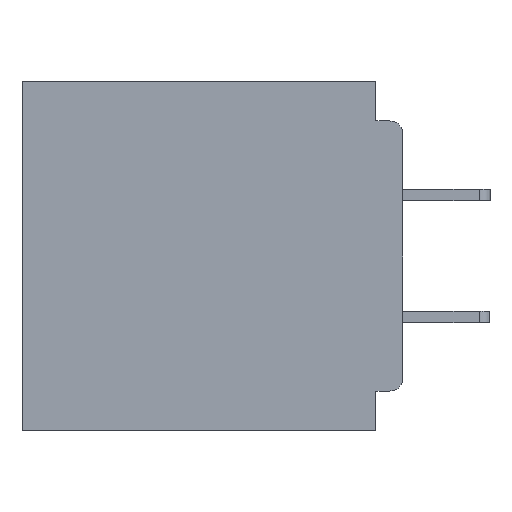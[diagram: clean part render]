
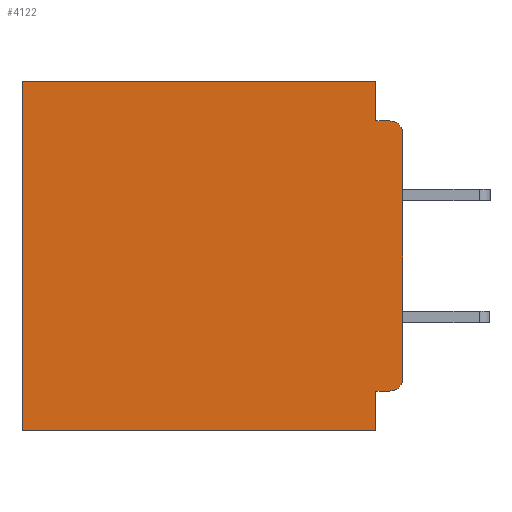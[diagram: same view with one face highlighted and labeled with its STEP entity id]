
A CAD part, left-side view. The second image highlights one B-rep face of the part: STEP entity #4122.
In plain terms, the highlighted planar face has unit normal (-1, 0, 0).
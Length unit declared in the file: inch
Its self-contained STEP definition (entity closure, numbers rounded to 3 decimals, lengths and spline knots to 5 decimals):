
#829 = DIRECTION ( 'NONE',  ( 0., 0., -1. ) ) ;
#1497 = EDGE_CURVE ( 'NONE', #15435, #42395, #46461, .T. ) ;
#2104 = VERTEX_POINT ( 'NONE', #49662 ) ;
#2227 = CARTESIAN_POINT ( 'NONE',  ( 0.3, 0., -0.4 ) ) ;
#4122 = ADVANCED_FACE ( 'NONE', ( #38104 ), #5828, .F. ) ;
#4322 = CARTESIAN_POINT ( 'NONE',  ( 0.3, 0., -0.045 ) ) ;
#4369 = VECTOR ( 'NONE', #24599, 39.37008 ) ;
#4774 = LINE ( 'NONE', #38134, #16652 ) ;
#5394 = CARTESIAN_POINT ( 'NONE',  ( 0.3, 0., -0.4 ) ) ;
#5728 = DIRECTION ( 'NONE',  ( 0., 0., -1. ) ) ;
#5828 = PLANE ( 'NONE',  #31712 ) ;
#6234 = LINE ( 'NONE', #2227, #47389 ) ;
#6326 = VECTOR ( 'NONE', #12518, 39.37008 ) ;
#9320 = CARTESIAN_POINT ( 'NONE',  ( 0.3, 0., -0.4 ) ) ;
#9468 = ORIENTED_EDGE ( 'NONE', *, *, #34428, .T. ) ;
#10215 = EDGE_CURVE ( 'NONE', #11888, #2104, #6234, .T. ) ;
#10502 = LINE ( 'NONE', #5394, #30413 ) ;
#10671 = ORIENTED_EDGE ( 'NONE', *, *, #44142, .F. ) ;
#11549 = LINE ( 'NONE', #29587, #42146 ) ;
#11888 = VERTEX_POINT ( 'NONE', #24225 ) ;
#12071 = DIRECTION ( 'NONE',  ( 1., 0., 0. ) ) ;
#12518 = DIRECTION ( 'NONE',  ( 0., -1., 0. ) ) ;
#12870 = LINE ( 'NONE', #25888, #43492 ) ;
#13113 = ORIENTED_EDGE ( 'NONE', *, *, #10215, .F. ) ;
#13621 = DIRECTION ( 'NONE',  ( -1., 0., 0. ) ) ;
#13748 = ORIENTED_EDGE ( 'NONE', *, *, #50404, .T. ) ;
#14143 = CARTESIAN_POINT ( 'NONE',  ( 0.3, 0., 0. ) ) ;
#14202 = DIRECTION ( 'NONE',  ( 0., 0., -1. ) ) ;
#14227 = AXIS2_PLACEMENT_3D ( 'NONE', #37553, #13621, #41594 ) ;
#14376 = ORIENTED_EDGE ( 'NONE', *, *, #23492, .T. ) ;
#14656 = VECTOR ( 'NONE', #24573, 39.37008 ) ;
#15435 = VERTEX_POINT ( 'NONE', #38321 ) ;
#16652 = VECTOR ( 'NONE', #14202, 39.37008 ) ;
#18166 = DIRECTION ( 'NONE',  ( 0., 1., 0. ) ) ;
#18540 = VERTEX_POINT ( 'NONE', #19101 ) ;
#19101 = CARTESIAN_POINT ( 'NONE',  ( 0.3, 0.015, -0.045 ) ) ;
#19193 = AXIS2_PLACEMENT_3D ( 'NONE', #48578, #24696, #829 ) ;
#19322 = ORIENTED_EDGE ( 'NONE', *, *, #1497, .T. ) ;
#21391 = CARTESIAN_POINT ( 'NONE',  ( 0.3, 0.031, -0.045 ) ) ;
#21420 = VERTEX_POINT ( 'NONE', #49924 ) ;
#23492 = EDGE_CURVE ( 'NONE', #42395, #2104, #11549, .T. ) ;
#23635 = VERTEX_POINT ( 'NONE', #38523 ) ;
#24225 = CARTESIAN_POINT ( 'NONE',  ( 0.3, 0.031, -0.4 ) ) ;
#24573 = DIRECTION ( 'NONE',  ( 0., 1., 0. ) ) ;
#24599 = DIRECTION ( 'NONE',  ( 0., 1., 0. ) ) ;
#24696 = DIRECTION ( 'NONE',  ( -1., 0., 0. ) ) ;
#24853 = ORIENTED_EDGE ( 'NONE', *, *, #39271, .F. ) ;
#25574 = LINE ( 'NONE', #44505, #4369 ) ;
#25860 = VERTEX_POINT ( 'NONE', #21391 ) ;
#25888 = CARTESIAN_POINT ( 'NONE',  ( 0.3, 0.031, 0. ) ) ;
#26818 = ORIENTED_EDGE ( 'NONE', *, *, #33888, .F. ) ;
#28043 = CARTESIAN_POINT ( 'NONE',  ( 0.3, 0., -0.34 ) ) ;
#28608 = ORIENTED_EDGE ( 'NONE', *, *, #43178, .F. ) ;
#29587 = CARTESIAN_POINT ( 'NONE',  ( 0.3, 0.437, -0.4 ) ) ;
#30413 = VECTOR ( 'NONE', #37324, 39.37008 ) ;
#31712 = AXIS2_PLACEMENT_3D ( 'NONE', #9320, #12071, #44938 ) ;
#33136 = EDGE_CURVE ( 'NONE', #47027, #35578, #10502, .T. ) ;
#33888 = EDGE_CURVE ( 'NONE', #21420, #11888, #4774, .T. ) ;
#34428 = EDGE_CURVE ( 'NONE', #23635, #35578, #42207, .T. ) ;
#35578 = VERTEX_POINT ( 'NONE', #28043 ) ;
#37324 = DIRECTION ( 'NONE',  ( 0., 0., -1. ) ) ;
#37553 = CARTESIAN_POINT ( 'NONE',  ( 0.3, 0.015, -0.34 ) ) ;
#38104 = FACE_OUTER_BOUND ( 'NONE', #39883, .T. ) ;
#38134 = CARTESIAN_POINT ( 'NONE',  ( 0.3, 0.031, -0.4 ) ) ;
#38165 = LINE ( 'NONE', #4322, #6326 ) ;
#38321 = CARTESIAN_POINT ( 'NONE',  ( 0.3, 0.031, 0. ) ) ;
#38523 = CARTESIAN_POINT ( 'NONE',  ( 0.3, 0.015, -0.355 ) ) ;
#39271 = EDGE_CURVE ( 'NONE', #15435, #25860, #12870, .T. ) ;
#39883 = EDGE_LOOP ( 'NONE', ( #41140, #13748, #28608, #24853, #19322, #14376, #13113, #26818, #10671, #9468 ) ) ;
#41140 = ORIENTED_EDGE ( 'NONE', *, *, #33136, .F. ) ;
#41594 = DIRECTION ( 'NONE',  ( 0., 0., -1. ) ) ;
#42146 = VECTOR ( 'NONE', #5728, 39.37008 ) ;
#42207 = CIRCLE ( 'NONE', #14227, 0.015 ) ;
#42395 = VERTEX_POINT ( 'NONE', #43337 ) ;
#43178 = EDGE_CURVE ( 'NONE', #25860, #18540, #38165, .T. ) ;
#43337 = CARTESIAN_POINT ( 'NONE',  ( 0.3, 0.437, 0. ) ) ;
#43492 = VECTOR ( 'NONE', #45953, 39.37008 ) ;
#44142 = EDGE_CURVE ( 'NONE', #23635, #21420, #25574, .T. ) ;
#44341 = CARTESIAN_POINT ( 'NONE',  ( 0.3, 0., -0.06 ) ) ;
#44505 = CARTESIAN_POINT ( 'NONE',  ( 0.3, 0., -0.355 ) ) ;
#44938 = DIRECTION ( 'NONE',  ( 0., 0., -1. ) ) ;
#45953 = DIRECTION ( 'NONE',  ( 0., 0., -1. ) ) ;
#46461 = LINE ( 'NONE', #14143, #14656 ) ;
#47027 = VERTEX_POINT ( 'NONE', #44341 ) ;
#47389 = VECTOR ( 'NONE', #18166, 39.37008 ) ;
#48578 = CARTESIAN_POINT ( 'NONE',  ( 0.3, 0.015, -0.06 ) ) ;
#49662 = CARTESIAN_POINT ( 'NONE',  ( 0.3, 0.437, -0.4 ) ) ;
#49924 = CARTESIAN_POINT ( 'NONE',  ( 0.3, 0.031, -0.355 ) ) ;
#50404 = EDGE_CURVE ( 'NONE', #47027, #18540, #51267, .T. ) ;
#51267 = CIRCLE ( 'NONE', #19193, 0.015 ) ;
